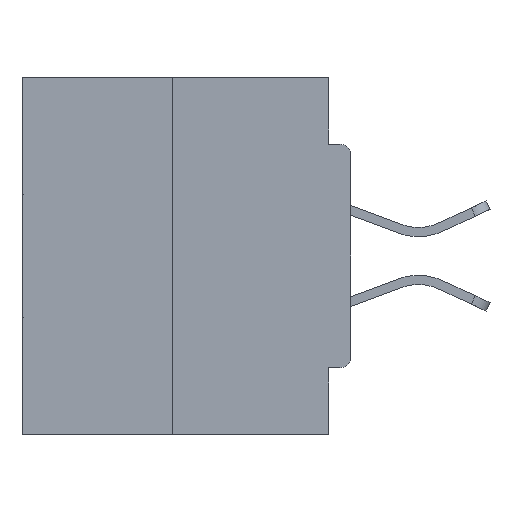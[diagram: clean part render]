
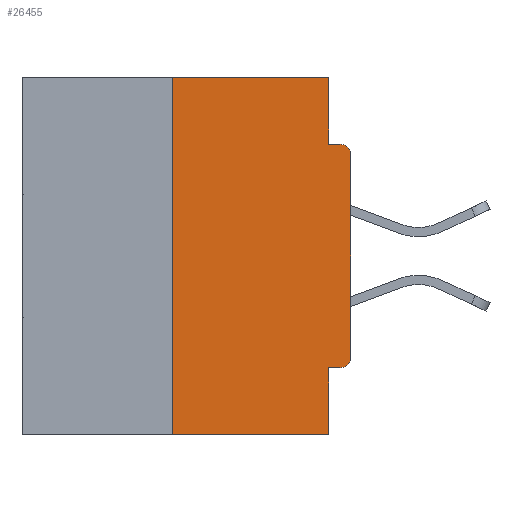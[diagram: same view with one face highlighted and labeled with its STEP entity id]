
A CAD part, left-side view. The second image highlights one B-rep face of the part: STEP entity #26455.
In plain terms, the highlighted planar face has unit normal (-1, 0, 0).
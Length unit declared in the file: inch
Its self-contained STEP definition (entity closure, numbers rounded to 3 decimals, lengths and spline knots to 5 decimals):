
#38 = CARTESIAN_POINT ( 'NONE',  ( 0., 0.015, -0.1085 ) ) ;
#60 = LINE ( 'NONE', #7873, #27695 ) ;
#446 = ORIENTED_EDGE ( 'NONE', *, *, #7102, .F. ) ;
#691 = VERTEX_POINT ( 'NONE', #31799 ) ;
#823 = CARTESIAN_POINT ( 'NONE',  ( 0., 0.25, 0. ) ) ;
#1247 = EDGE_CURVE ( 'NONE', #22680, #16818, #1694, .T. ) ;
#1694 = LINE ( 'NONE', #4930, #25012 ) ;
#2503 = ORIENTED_EDGE ( 'NONE', *, *, #27047, .T. ) ;
#3515 = VERTEX_POINT ( 'NONE', #12682 ) ;
#4130 = FACE_OUTER_BOUND ( 'NONE', #33007, .T. ) ;
#4930 = CARTESIAN_POINT ( 'NONE',  ( 0., 0., -0.0935 ) ) ;
#5867 = CARTESIAN_POINT ( 'NONE',  ( 0., 0., 0. ) ) ;
#6270 = ORIENTED_EDGE ( 'NONE', *, *, #36136, .T. ) ;
#6783 = DIRECTION ( 'NONE',  ( 0., 0., 1. ) ) ;
#6902 = VERTEX_POINT ( 'NONE', #34599 ) ;
#7102 = EDGE_CURVE ( 'NONE', #3515, #22559, #60, .T. ) ;
#7873 = CARTESIAN_POINT ( 'NONE',  ( 0., 0., -0.4065 ) ) ;
#8392 = CARTESIAN_POINT ( 'NONE',  ( 0., 0.46, 0. ) ) ;
#8468 = VECTOR ( 'NONE', #16284, 39.37008 ) ;
#8629 = DIRECTION ( 'NONE',  ( 0., -1., 0. ) ) ;
#9049 = DIRECTION ( 'NONE',  ( -1., 0., 0. ) ) ;
#9416 = LINE ( 'NONE', #13191, #32249 ) ;
#10077 = CARTESIAN_POINT ( 'NONE',  ( 0., 0., -0.1085 ) ) ;
#10418 = LINE ( 'NONE', #19209, #8468 ) ;
#10992 = ORIENTED_EDGE ( 'NONE', *, *, #1247, .F. ) ;
#11592 = AXIS2_PLACEMENT_3D ( 'NONE', #14171, #23775, #20553 ) ;
#12225 = CIRCLE ( 'NONE', #31257, 0.015 ) ;
#12233 = CARTESIAN_POINT ( 'NONE',  ( 0., 0.25, 0. ) ) ;
#12682 = CARTESIAN_POINT ( 'NONE',  ( 0., 0.015, -0.4065 ) ) ;
#12697 = AXIS2_PLACEMENT_3D ( 'NONE', #38, #9049, #30603 ) ;
#13131 = DIRECTION ( 'NONE',  ( 0., 0., -1. ) ) ;
#13191 = CARTESIAN_POINT ( 'NONE',  ( 0., 0.46, -0.5 ) ) ;
#13197 = VERTEX_POINT ( 'NONE', #10077 ) ;
#14171 = CARTESIAN_POINT ( 'NONE',  ( 0., 0.46, 0. ) ) ;
#15262 = EDGE_CURVE ( 'NONE', #22559, #32365, #10418, .T. ) ;
#15800 = ORIENTED_EDGE ( 'NONE', *, *, #29238, .F. ) ;
#15930 = VERTEX_POINT ( 'NONE', #12233 ) ;
#16284 = DIRECTION ( 'NONE',  ( 0., 0., -1. ) ) ;
#16397 = LINE ( 'NONE', #8392, #26926 ) ;
#16818 = VERTEX_POINT ( 'NONE', #34625 ) ;
#16863 = DIRECTION ( 'NONE',  ( 0., 1., 0. ) ) ;
#17150 = DIRECTION ( 'NONE',  ( 0., -1., 0. ) ) ;
#19209 = CARTESIAN_POINT ( 'NONE',  ( 0., 0.031, -0.5 ) ) ;
#20156 = PLANE ( 'NONE',  #11592 ) ;
#20553 = DIRECTION ( 'NONE',  ( 0., 0., -1. ) ) ;
#21131 = CARTESIAN_POINT ( 'NONE',  ( 0., 0.031, -0.4065 ) ) ;
#22169 = ORIENTED_EDGE ( 'NONE', *, *, #34210, .F. ) ;
#22219 = CARTESIAN_POINT ( 'NONE',  ( 0., 0.25, -0.5 ) ) ;
#22559 = VERTEX_POINT ( 'NONE', #21131 ) ;
#22680 = VERTEX_POINT ( 'NONE', #33907 ) ;
#22884 = VECTOR ( 'NONE', #13131, 39.37008 ) ;
#23299 = ORIENTED_EDGE ( 'NONE', *, *, #31089, .T. ) ;
#23749 = CARTESIAN_POINT ( 'NONE',  ( 0., 0.031, -0.5 ) ) ;
#23775 = DIRECTION ( 'NONE',  ( 1., 0., 0. ) ) ;
#23887 = VECTOR ( 'NONE', #27022, 39.37008 ) ;
#24004 = CIRCLE ( 'NONE', #12697, 0.015 ) ;
#25012 = VECTOR ( 'NONE', #8629, 39.37008 ) ;
#25373 = ORIENTED_EDGE ( 'NONE', *, *, #30005, .T. ) ;
#25681 = VECTOR ( 'NONE', #6783, 39.37008 ) ;
#26166 = EDGE_CURVE ( 'NONE', #36905, #15930, #30878, .T. ) ;
#26455 = ADVANCED_FACE ( 'NONE', ( #4130 ), #20156, .F. ) ;
#26926 = VECTOR ( 'NONE', #17150, 39.37008 ) ;
#27022 = DIRECTION ( 'NONE',  ( 0., 0., 1. ) ) ;
#27029 = DIRECTION ( 'NONE',  ( 0., 0., -1. ) ) ;
#27047 = EDGE_CURVE ( 'NONE', #3515, #6902, #12225, .T. ) ;
#27695 = VECTOR ( 'NONE', #16863, 39.37008 ) ;
#29238 = EDGE_CURVE ( 'NONE', #15930, #691, #16397, .T. ) ;
#30005 = EDGE_CURVE ( 'NONE', #13197, #16818, #24004, .T. ) ;
#30068 = DIRECTION ( 'NONE',  ( -1., 0., 0. ) ) ;
#30523 = DIRECTION ( 'NONE',  ( 0., -1., 0. ) ) ;
#30603 = DIRECTION ( 'NONE',  ( 0., 0., -1. ) ) ;
#30878 = LINE ( 'NONE', #823, #25681 ) ;
#31089 = EDGE_CURVE ( 'NONE', #6902, #13197, #31955, .T. ) ;
#31257 = AXIS2_PLACEMENT_3D ( 'NONE', #36538, #30068, #27029 ) ;
#31388 = CARTESIAN_POINT ( 'NONE',  ( 0., 0.031, 0. ) ) ;
#31799 = CARTESIAN_POINT ( 'NONE',  ( 0., 0.031, 0. ) ) ;
#31955 = LINE ( 'NONE', #5867, #23887 ) ;
#32249 = VECTOR ( 'NONE', #30523, 39.37008 ) ;
#32365 = VERTEX_POINT ( 'NONE', #23749 ) ;
#32402 = LINE ( 'NONE', #31388, #22884 ) ;
#32731 = ORIENTED_EDGE ( 'NONE', *, *, #15262, .F. ) ;
#33007 = EDGE_LOOP ( 'NONE', ( #15800, #37150, #6270, #32731, #446, #2503, #23299, #25373, #10992, #22169 ) ) ;
#33907 = CARTESIAN_POINT ( 'NONE',  ( 0., 0.031, -0.0935 ) ) ;
#34210 = EDGE_CURVE ( 'NONE', #691, #22680, #32402, .T. ) ;
#34599 = CARTESIAN_POINT ( 'NONE',  ( 0., 0., -0.3915 ) ) ;
#34625 = CARTESIAN_POINT ( 'NONE',  ( 0., 0.015, -0.0935 ) ) ;
#36136 = EDGE_CURVE ( 'NONE', #36905, #32365, #9416, .T. ) ;
#36538 = CARTESIAN_POINT ( 'NONE',  ( 0., 0.015, -0.3915 ) ) ;
#36905 = VERTEX_POINT ( 'NONE', #22219 ) ;
#37150 = ORIENTED_EDGE ( 'NONE', *, *, #26166, .F. ) ;
